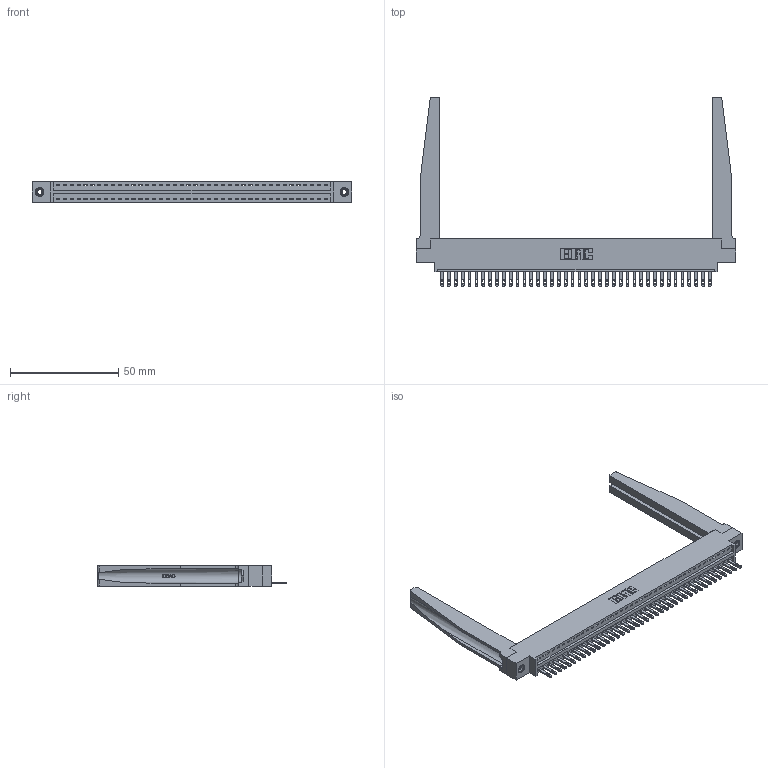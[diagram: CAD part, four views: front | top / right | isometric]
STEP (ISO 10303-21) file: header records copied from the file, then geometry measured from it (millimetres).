
FILE_DESCRIPTION (( 'STEP AP203' ), '1' );
FILE_NAME ('346-040-500-678.STEP', '2022-05-07T08:34:26', ( '' ), ( '' ), 'SwSTEP 2.0', 'SolidWorks 2020', '' );
FILE_SCHEMA (( 'CONFIG_CONTROL_DESIGN' ));
Length unit declared in the file: inch
Products named in the file (5): 346-040-500-678; 346 Part_0.170 Offset - 0.156 Dia-TH; 345-292-001_345-293-100; 346-220-078_345-220-078; 345-250-001_345-250-001-102
Assembly tree (45 placements, depth 2):
  346-040-500-678
    346 Part_0.170 Offset - 0.156 Dia-TH
    345-292-001_345-293-100  x40
    346-220-078_345-220-078  x2
    345-250-001_345-250-001-102  x2
Bounding box: 147.57 x 87.12 x 9.4 mm (x, y, z)
Volume: 20873.2 mm3; surface area: 24258 mm2
Topology: 45 solids, 45 shells, 2534 faces, 7705 edges, 5126 vertices
Faces by surface type: plane 1596, cylinder 886, bspline 36, cone 12, torus 4
Entity records: 30320 total; most frequent: CARTESIAN_POINT 6113, ORIENTED_EDGE 4974, DIRECTION 4381, EDGE_CURVE 2487, LINE 2097, VECTOR 2097, VERTEX_POINT 1652, AXIS2_PLACEMENT_3D 1142
